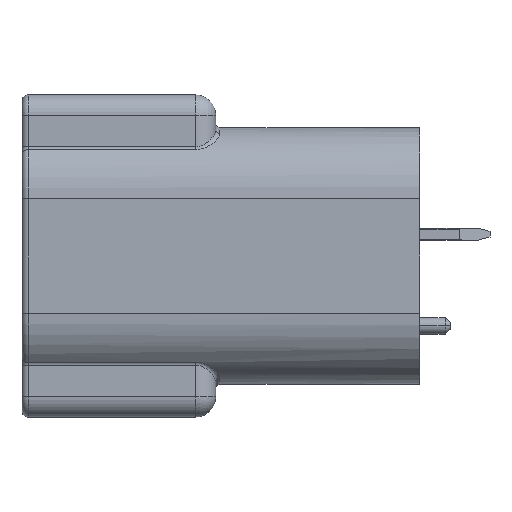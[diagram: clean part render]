
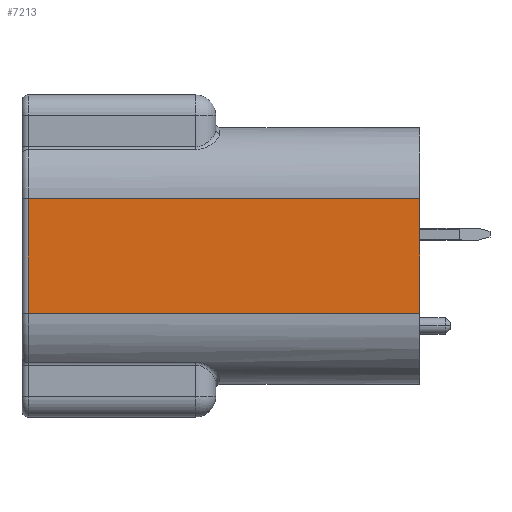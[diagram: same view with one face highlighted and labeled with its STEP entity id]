
A CAD part, left-side view. The second image highlights one B-rep face of the part: STEP entity #7213.
In plain terms, the highlighted planar face has unit normal (-1, 0, 0).
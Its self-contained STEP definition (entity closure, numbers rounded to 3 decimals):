
#101 = VECTOR ( 'NONE', #5137, 1000. ) ;
#1087 = VECTOR ( 'NONE', #2810, 1000. ) ;
#1156 = VERTEX_POINT ( 'NONE', #8927 ) ;
#1253 = LINE ( 'NONE', #6654, #5237 ) ;
#1460 = CARTESIAN_POINT ( 'NONE',  ( -6.4, -5.75, -2.8 ) ) ;
#1512 = EDGE_CURVE ( 'NONE', #8415, #7181, #8624, .T. ) ;
#1843 = CARTESIAN_POINT ( 'NONE',  ( -6.4, -5.75, 2.8 ) ) ;
#1960 = CARTESIAN_POINT ( 'NONE',  ( -6.4, -5.75, 2.8 ) ) ;
#2073 = DIRECTION ( 'NONE',  ( 0., 0., 1. ) ) ;
#2218 = LINE ( 'NONE', #6026, #6575 ) ;
#2255 = EDGE_CURVE ( 'NONE', #1156, #8415, #2218, .T. ) ;
#2539 = CARTESIAN_POINT ( 'NONE',  ( -6.4, 13.45, -2.8 ) ) ;
#2791 = AXIS2_PLACEMENT_3D ( 'NONE', #6829, #3919, #6057 ) ;
#2810 = DIRECTION ( 'NONE',  ( 0., 1., 0. ) ) ;
#2847 = EDGE_CURVE ( 'NONE', #3446, #7181, #1253, .T. ) ;
#3446 = VERTEX_POINT ( 'NONE', #2539 ) ;
#3825 = FACE_OUTER_BOUND ( 'NONE', #4016, .T. ) ;
#3919 = DIRECTION ( 'NONE',  ( -1., 0., 0. ) ) ;
#4016 = EDGE_LOOP ( 'NONE', ( #8695, #6170, #4527, #7509 ) ) ;
#4527 = ORIENTED_EDGE ( 'NONE', *, *, #2255, .T. ) ;
#5137 = DIRECTION ( 'NONE',  ( 0., 1., 0. ) ) ;
#5237 = VECTOR ( 'NONE', #2073, 1000. ) ;
#5797 = LINE ( 'NONE', #1460, #1087 ) ;
#6026 = CARTESIAN_POINT ( 'NONE',  ( -6.4, -5.75, -2.8 ) ) ;
#6057 = DIRECTION ( 'NONE',  ( 0., 0., -1. ) ) ;
#6170 = ORIENTED_EDGE ( 'NONE', *, *, #7921, .F. ) ;
#6575 = VECTOR ( 'NONE', #7375, 1000. ) ;
#6654 = CARTESIAN_POINT ( 'NONE',  ( -6.4, 13.45, -2.8 ) ) ;
#6829 = CARTESIAN_POINT ( 'NONE',  ( -6.4, 13.75, 6.3 ) ) ;
#6873 = CARTESIAN_POINT ( 'NONE',  ( -6.4, 13.45, 2.8 ) ) ;
#7181 = VERTEX_POINT ( 'NONE', #6873 ) ;
#7213 = ADVANCED_FACE ( 'NONE', ( #3825 ), #7504, .T. ) ;
#7375 = DIRECTION ( 'NONE',  ( 0., 0., 1. ) ) ;
#7504 = PLANE ( 'NONE',  #2791 ) ;
#7509 = ORIENTED_EDGE ( 'NONE', *, *, #1512, .T. ) ;
#7921 = EDGE_CURVE ( 'NONE', #1156, #3446, #5797, .T. ) ;
#8415 = VERTEX_POINT ( 'NONE', #1843 ) ;
#8624 = LINE ( 'NONE', #1960, #101 ) ;
#8695 = ORIENTED_EDGE ( 'NONE', *, *, #2847, .F. ) ;
#8927 = CARTESIAN_POINT ( 'NONE',  ( -6.4, -5.75, -2.8 ) ) ;
